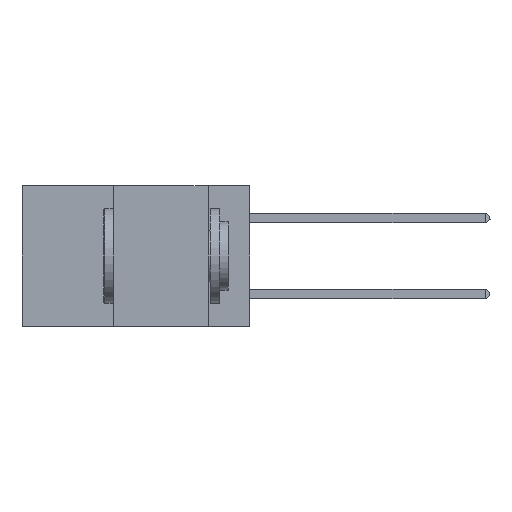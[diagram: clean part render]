
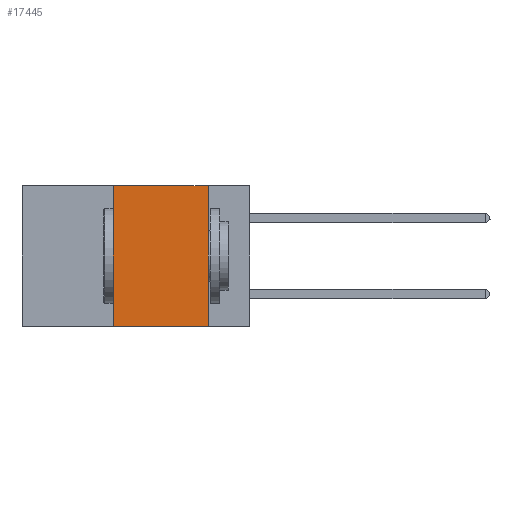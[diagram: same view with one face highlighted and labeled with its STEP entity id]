
A CAD part, left-side view. The second image highlights one B-rep face of the part: STEP entity #17445.
In plain terms, the highlighted planar face has unit normal (-1, 0, 0).
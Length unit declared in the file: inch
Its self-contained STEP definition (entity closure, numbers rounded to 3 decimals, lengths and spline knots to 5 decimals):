
#153 = VECTOR ( 'NONE', #13275, 39.37008 ) ;
#1262 = VECTOR ( 'NONE', #23030, 39.37008 ) ;
#2593 = DIRECTION ( 'NONE',  ( 0., -1., 0. ) ) ;
#2628 = CARTESIAN_POINT ( 'NONE',  ( 0., 0.11, -0.37 ) ) ;
#2808 = CARTESIAN_POINT ( 'NONE',  ( 0., 0.36, -0.37 ) ) ;
#3172 = VERTEX_POINT ( 'NONE', #2628 ) ;
#3360 = EDGE_CURVE ( 'NONE', #13520, #3172, #23305, .T. ) ;
#5486 = PLANE ( 'NONE',  #14170 ) ;
#6483 = CARTESIAN_POINT ( 'NONE',  ( 0., 0.6, 0. ) ) ;
#7865 = ORIENTED_EDGE ( 'NONE', *, *, #8198, .T. ) ;
#8066 = ORIENTED_EDGE ( 'NONE', *, *, #12103, .F. ) ;
#8198 = EDGE_CURVE ( 'NONE', #20459, #3172, #20053, .T. ) ;
#8484 = LINE ( 'NONE', #9537, #153 ) ;
#9537 = CARTESIAN_POINT ( 'NONE',  ( 0., 0.36, 0. ) ) ;
#9556 = DIRECTION ( 'NONE',  ( 1., 0., 0. ) ) ;
#9633 = DIRECTION ( 'NONE',  ( 0., 0., -1. ) ) ;
#10649 = FACE_OUTER_BOUND ( 'NONE', #15537, .T. ) ;
#11602 = LINE ( 'NONE', #6483, #24406 ) ;
#12103 = EDGE_CURVE ( 'NONE', #17098, #13520, #11602, .T. ) ;
#12414 = CARTESIAN_POINT ( 'NONE',  ( 0., 0.6, -0.37 ) ) ;
#12839 = ORIENTED_EDGE ( 'NONE', *, *, #17994, .F. ) ;
#12924 = ORIENTED_EDGE ( 'NONE', *, *, #3360, .F. ) ;
#13275 = DIRECTION ( 'NONE',  ( 0., 0., 1. ) ) ;
#13520 = VERTEX_POINT ( 'NONE', #17745 ) ;
#14170 = AXIS2_PLACEMENT_3D ( 'NONE', #24861, #9556, #9633 ) ;
#15460 = VECTOR ( 'NONE', #18516, 39.37008 ) ;
#15537 = EDGE_LOOP ( 'NONE', ( #12924, #8066, #12839, #7865 ) ) ;
#15777 = CARTESIAN_POINT ( 'NONE',  ( 0., 0.36, 0. ) ) ;
#17098 = VERTEX_POINT ( 'NONE', #15777 ) ;
#17445 = ADVANCED_FACE ( 'NONE', ( #10649 ), #5486, .F. ) ;
#17745 = CARTESIAN_POINT ( 'NONE',  ( 0., 0.11, 0. ) ) ;
#17994 = EDGE_CURVE ( 'NONE', #20459, #17098, #8484, .T. ) ;
#18516 = DIRECTION ( 'NONE',  ( 0., -1., 0. ) ) ;
#20053 = LINE ( 'NONE', #12414, #15460 ) ;
#20459 = VERTEX_POINT ( 'NONE', #2808 ) ;
#21152 = CARTESIAN_POINT ( 'NONE',  ( 0., 0.11, 0. ) ) ;
#23030 = DIRECTION ( 'NONE',  ( 0., 0., -1. ) ) ;
#23305 = LINE ( 'NONE', #21152, #1262 ) ;
#24406 = VECTOR ( 'NONE', #2593, 39.37008 ) ;
#24861 = CARTESIAN_POINT ( 'NONE',  ( 0., 0.6, 0. ) ) ;
